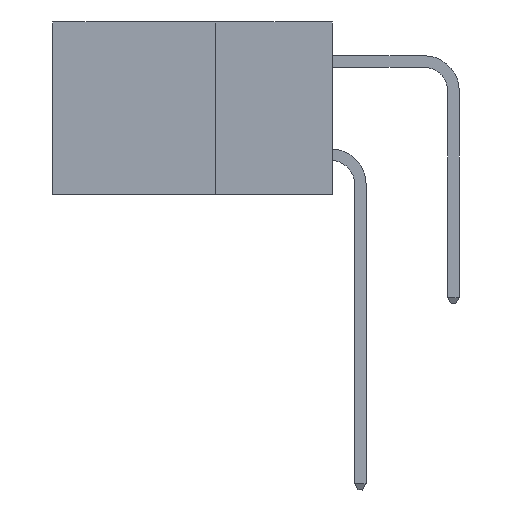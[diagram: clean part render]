
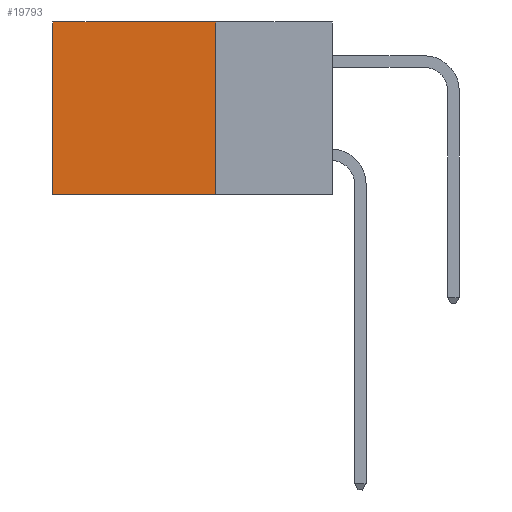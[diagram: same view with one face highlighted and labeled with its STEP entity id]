
A CAD part, left-side view. The second image highlights one B-rep face of the part: STEP entity #19793.
In plain terms, the highlighted planar face has unit normal (-1, 0, 0).
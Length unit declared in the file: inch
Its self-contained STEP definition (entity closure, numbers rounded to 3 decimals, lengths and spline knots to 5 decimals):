
#780 = CARTESIAN_POINT ( 'NONE',  ( 0.298, 0.25, -0.37 ) ) ;
#1956 = FACE_OUTER_BOUND ( 'NONE', #25198, .T. ) ;
#2131 = VERTEX_POINT ( 'NONE', #16135 ) ;
#2235 = VECTOR ( 'NONE', #23998, 39.37008 ) ;
#2781 = EDGE_CURVE ( 'NONE', #15111, #19391, #24293, .T. ) ;
#4243 = ORIENTED_EDGE ( 'NONE', *, *, #25437, .T. ) ;
#5482 = CARTESIAN_POINT ( 'NONE',  ( 0.298, 0.25, 0. ) ) ;
#5701 = LINE ( 'NONE', #23626, #9709 ) ;
#6289 = CARTESIAN_POINT ( 'NONE',  ( 0.298, 0.25, 0. ) ) ;
#6564 = DIRECTION ( 'NONE',  ( 0., 0., -1. ) ) ;
#8167 = ORIENTED_EDGE ( 'NONE', *, *, #23801, .F. ) ;
#9319 = CARTESIAN_POINT ( 'NONE',  ( 0.298, 0.25, 0. ) ) ;
#9631 = LINE ( 'NONE', #15415, #2235 ) ;
#9709 = VECTOR ( 'NONE', #6564, 39.37008 ) ;
#13364 = CARTESIAN_POINT ( 'NONE',  ( 0.298, 0.25, 0. ) ) ;
#13447 = DIRECTION ( 'NONE',  ( 0., 1., 0. ) ) ;
#13633 = DIRECTION ( 'NONE',  ( 0., 0., -1. ) ) ;
#15111 = VERTEX_POINT ( 'NONE', #5482 ) ;
#15415 = CARTESIAN_POINT ( 'NONE',  ( 0.298, 0.25, -0.37 ) ) ;
#15974 = LINE ( 'NONE', #6289, #16956 ) ;
#16135 = CARTESIAN_POINT ( 'NONE',  ( 0.298, 0.6, -0.37 ) ) ;
#16278 = VERTEX_POINT ( 'NONE', #780 ) ;
#16956 = VECTOR ( 'NONE', #23485, 39.37008 ) ;
#18039 = PLANE ( 'NONE',  #25947 ) ;
#19391 = VERTEX_POINT ( 'NONE', #22398 ) ;
#19793 = ADVANCED_FACE ( 'NONE', ( #1956 ), #18039, .F. ) ;
#22301 = DIRECTION ( 'NONE',  ( 1., 0., 0. ) ) ;
#22398 = CARTESIAN_POINT ( 'NONE',  ( 0.298, 0.6, 0. ) ) ;
#22590 = VECTOR ( 'NONE', #13447, 39.37008 ) ;
#22857 = ORIENTED_EDGE ( 'NONE', *, *, #23544, .F. ) ;
#23485 = DIRECTION ( 'NONE',  ( 0., 0., -1. ) ) ;
#23544 = EDGE_CURVE ( 'NONE', #16278, #2131, #9631, .T. ) ;
#23626 = CARTESIAN_POINT ( 'NONE',  ( 0.298, 0.6, 0. ) ) ;
#23801 = EDGE_CURVE ( 'NONE', #15111, #16278, #15974, .T. ) ;
#23998 = DIRECTION ( 'NONE',  ( 0., 1., 0. ) ) ;
#24293 = LINE ( 'NONE', #9319, #22590 ) ;
#25198 = EDGE_LOOP ( 'NONE', ( #4243, #22857, #8167, #25374 ) ) ;
#25374 = ORIENTED_EDGE ( 'NONE', *, *, #2781, .T. ) ;
#25437 = EDGE_CURVE ( 'NONE', #19391, #2131, #5701, .T. ) ;
#25947 = AXIS2_PLACEMENT_3D ( 'NONE', #13364, #22301, #13633 ) ;
